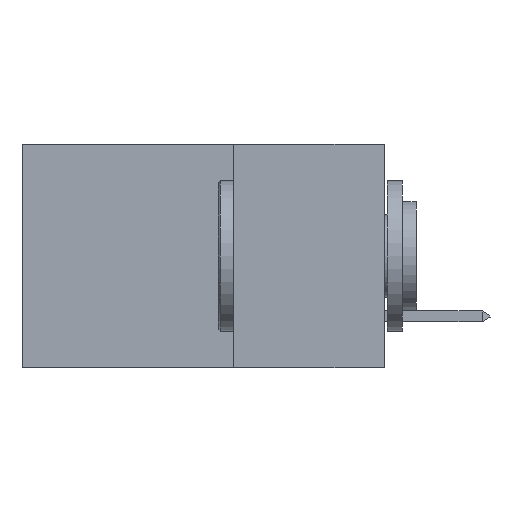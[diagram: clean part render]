
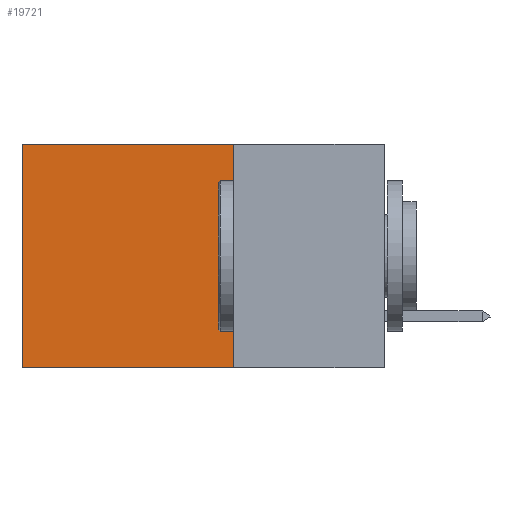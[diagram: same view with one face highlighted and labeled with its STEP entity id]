
A CAD part, left-side view. The second image highlights one B-rep face of the part: STEP entity #19721.
In plain terms, the highlighted planar face has unit normal (-1, 0, 0).
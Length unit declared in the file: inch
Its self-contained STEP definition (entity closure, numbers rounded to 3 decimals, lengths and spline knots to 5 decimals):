
#706 = CARTESIAN_POINT ( 'NONE',  ( 0.2875, 0.25, 0. ) ) ;
#3959 = EDGE_CURVE ( 'NONE', #43981, #34471, #24497, .T. ) ;
#5852 = ORIENTED_EDGE ( 'NONE', *, *, #35837, .F. ) ;
#8960 = PLANE ( 'NONE',  #34156 ) ;
#9739 = EDGE_CURVE ( 'NONE', #16823, #30892, #19636, .T. ) ;
#10913 = EDGE_CURVE ( 'NONE', #34471, #30892, #35994, .T. ) ;
#11432 = DIRECTION ( 'NONE',  ( 0., 0., -1. ) ) ;
#11793 = LINE ( 'NONE', #31287, #14017 ) ;
#13859 = DIRECTION ( 'NONE',  ( 0., 0., -1. ) ) ;
#14017 = VECTOR ( 'NONE', #13859, 39.37008 ) ;
#15317 = ORIENTED_EDGE ( 'NONE', *, *, #9739, .F. ) ;
#15661 = CARTESIAN_POINT ( 'NONE',  ( 0.2875, 0.25, -0.37 ) ) ;
#16823 = VERTEX_POINT ( 'NONE', #19221 ) ;
#19221 = CARTESIAN_POINT ( 'NONE',  ( 0.2875, 0.25, -0.37 ) ) ;
#19636 = LINE ( 'NONE', #15661, #37184 ) ;
#19721 = ADVANCED_FACE ( 'NONE', ( #20937 ), #8960, .F. ) ;
#20937 = FACE_OUTER_BOUND ( 'NONE', #20997, .T. ) ;
#20965 = CARTESIAN_POINT ( 'NONE',  ( 0.2875, 0.6, 0. ) ) ;
#20997 = EDGE_LOOP ( 'NONE', ( #24460, #15317, #5852, #25648 ) ) ;
#23402 = VECTOR ( 'NONE', #35899, 39.37008 ) ;
#24408 = CARTESIAN_POINT ( 'NONE',  ( 0.2875, 0.25, 0. ) ) ;
#24460 = ORIENTED_EDGE ( 'NONE', *, *, #10913, .T. ) ;
#24497 = LINE ( 'NONE', #706, #23402 ) ;
#25648 = ORIENTED_EDGE ( 'NONE', *, *, #3959, .T. ) ;
#25969 = CARTESIAN_POINT ( 'NONE',  ( 0.2875, 0.6, 0. ) ) ;
#26194 = DIRECTION ( 'NONE',  ( 0., 0., -1. ) ) ;
#26627 = VECTOR ( 'NONE', #11432, 39.37008 ) ;
#30892 = VERTEX_POINT ( 'NONE', #36718 ) ;
#31055 = DIRECTION ( 'NONE',  ( 0., 1., 0. ) ) ;
#31287 = CARTESIAN_POINT ( 'NONE',  ( 0.2875, 0.25, 0. ) ) ;
#34156 = AXIS2_PLACEMENT_3D ( 'NONE', #36942, #37107, #26194 ) ;
#34471 = VERTEX_POINT ( 'NONE', #20965 ) ;
#35837 = EDGE_CURVE ( 'NONE', #43981, #16823, #11793, .T. ) ;
#35899 = DIRECTION ( 'NONE',  ( 0., 1., 0. ) ) ;
#35994 = LINE ( 'NONE', #25969, #26627 ) ;
#36718 = CARTESIAN_POINT ( 'NONE',  ( 0.2875, 0.6, -0.37 ) ) ;
#36942 = CARTESIAN_POINT ( 'NONE',  ( 0.2875, 0.25, 0. ) ) ;
#37107 = DIRECTION ( 'NONE',  ( 1., 0., 0. ) ) ;
#37184 = VECTOR ( 'NONE', #31055, 39.37008 ) ;
#43981 = VERTEX_POINT ( 'NONE', #24408 ) ;
